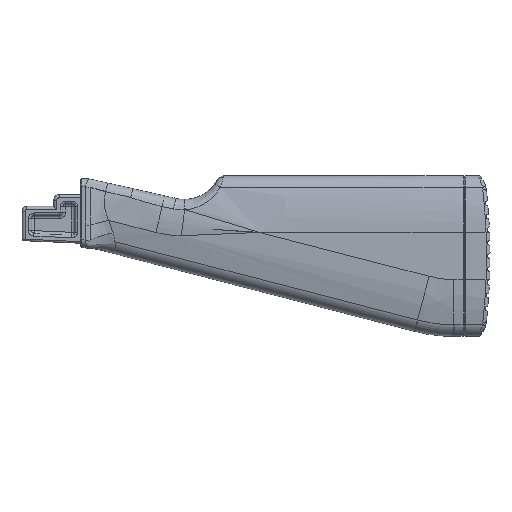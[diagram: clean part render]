
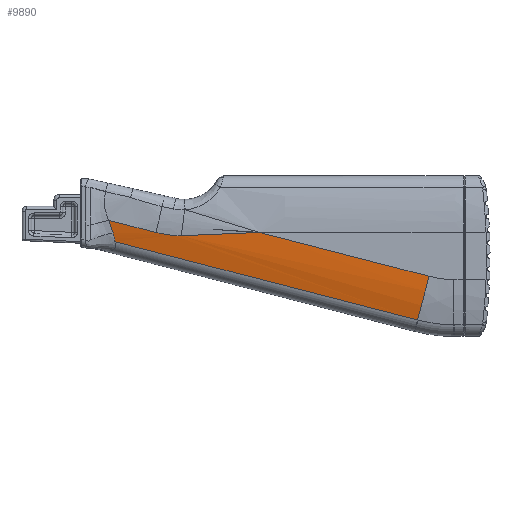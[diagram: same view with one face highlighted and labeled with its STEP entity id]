
A CAD part, left-side view. The second image highlights one B-rep face of the part: STEP entity #9890.
In plain terms, the highlighted cylindrical face has radius 115.186 mm (diameter 230.372 mm), a partial arc.
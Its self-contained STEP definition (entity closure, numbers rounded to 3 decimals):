
#368=LINE('',#16164,#820);
#514=LINE('',#30649,#966);
#820=VECTOR('',#11593,10.);
#966=VECTOR('',#12437,10.);
#1286=CYLINDRICAL_SURFACE('',#10739,115.186);
#1717=FACE_OUTER_BOUND('',#2382,.T.);
#2382=EDGE_LOOP('',(#7627,#7628,#7629,#7630,#7631,#7632,#7633,#7634,#7635));
#3047=CIRCLE('',#10731,115.186);
#3555=B_SPLINE_CURVE_WITH_KNOTS('',3,(#23032,#23033,#23034,#23035),
 .UNSPECIFIED.,.F.,.F.,(4,4),(5.073,6.041),
 .UNSPECIFIED.);
#3563=B_SPLINE_CURVE_WITH_KNOTS('',3,(#28936,#28937,#28938,#28939,#28940,
#28941),.UNSPECIFIED.,.F.,.F.,(4,2,4),(-12.142,-11.833,
-11.448),.UNSPECIFIED.);
#3585=B_SPLINE_CURVE_WITH_KNOTS('',3,(#30715,#30716,#30717,#30718),
 .UNSPECIFIED.,.F.,.F.,(4,4),(6.477,7.8),
 .UNSPECIFIED.);
#3586=B_SPLINE_CURVE_WITH_KNOTS('',3,(#30719,#30720,#30721,#30722),
 .UNSPECIFIED.,.F.,.F.,(4,4),(7.8,9.601),
 .UNSPECIFIED.);
#3587=B_SPLINE_CURVE_WITH_KNOTS('',3,(#30724,#30725,#30726,#30727,#30728,
#30729,#30730,#30731,#30732,#30733,#30734),.UNSPECIFIED.,.F.,.F.,(4,2,1,
1,1,1,1,4),(0.,0.006,0.975,
2.912,3.396,3.88,4.364,4.849),
 .UNSPECIFIED.);
#3588=B_SPLINE_CURVE_WITH_KNOTS('',3,(#30735,#30736,#30737,#30738,#30739,
#30740,#30741,#30742,#30743,#30744,#30745,#30746,#30747,#30748,#30749,#30750,
#30751,#30752,#30753,#30754,#30755,#30756,#30757),.UNSPECIFIED.,.F.,.F.,
(4,1,1,1,1,1,1,1,1,1,1,1,1,1,1,1,1,1,1,1,4),(4.849,4.888,
5.11,5.221,5.277,5.332,5.401,
5.459,5.518,5.576,5.635,5.694,
5.752,5.811,5.869,5.928,5.987,
6.045,6.158,6.265,6.477),
 .UNSPECIFIED.);
#3935=VERTEX_POINT('',#16161);
#3936=VERTEX_POINT('',#16163);
#4181=VERTEX_POINT('',#23029);
#4182=VERTEX_POINT('',#23031);
#4264=VERTEX_POINT('',#28923);
#4278=VERTEX_POINT('',#30640);
#4283=VERTEX_POINT('',#30713);
#4284=VERTEX_POINT('',#30714);
#4285=VERTEX_POINT('',#30723);
#4897=EDGE_CURVE('',#3936,#3935,#368,.T.);
#5303=EDGE_CURVE('',#4182,#4181,#3555,.T.);
#5439=EDGE_CURVE('',#4181,#4264,#3563,.T.);
#5468=EDGE_CURVE('',#4278,#3936,#3047,.T.);
#5469=EDGE_CURVE('',#4278,#4264,#514,.T.);
#5477=EDGE_CURVE('',#4283,#4284,#3585,.T.);
#5478=EDGE_CURVE('',#4284,#4182,#3586,.T.);
#5479=EDGE_CURVE('',#3935,#4285,#3587,.T.);
#5480=EDGE_CURVE('',#4285,#4283,#3588,.T.);
#7627=ORIENTED_EDGE('',*,*,#5477,.T.);
#7628=ORIENTED_EDGE('',*,*,#5478,.T.);
#7629=ORIENTED_EDGE('',*,*,#5303,.T.);
#7630=ORIENTED_EDGE('',*,*,#5439,.T.);
#7631=ORIENTED_EDGE('',*,*,#5469,.F.);
#7632=ORIENTED_EDGE('',*,*,#5468,.T.);
#7633=ORIENTED_EDGE('',*,*,#4897,.T.);
#7634=ORIENTED_EDGE('',*,*,#5479,.T.);
#7635=ORIENTED_EDGE('',*,*,#5480,.T.);
#9890=ADVANCED_FACE('',(#1717),#1286,.T.);
#10731=AXIS2_PLACEMENT_3D('',#30647,#12433,#12434);
#10739=AXIS2_PLACEMENT_3D('',#30712,#12451,#12452);
#11593=DIRECTION('',(0.,0.968,0.25));
#12433=DIRECTION('center_axis',(0.,0.967,0.253));
#12434=DIRECTION('ref_axis',(-0.949,0.08,-0.305));
#12437=DIRECTION('',(0.,0.968,0.25));
#12451=DIRECTION('center_axis',(0.,-0.968,-0.25));
#12452=DIRECTION('ref_axis',(-0.949,0.079,-0.305));
#16161=CARTESIAN_POINT('',(84.25,-573.566,96.326));
#16163=CARTESIAN_POINT('',(84.25,-681.487,68.407));
#16164=CARTESIAN_POINT('',(84.25,-681.381,68.434));
#23029=CARTESIAN_POINT('',(86.683,-480.14,96.168));
#23031=CARTESIAN_POINT('',(85.452,-477.378,104.065));
#23032=CARTESIAN_POINT('Ctrl Pts',(85.452,-477.378,104.065));
#23033=CARTESIAN_POINT('Ctrl Pts',(85.795,-478.261,101.405));
#23034=CARTESIAN_POINT('Ctrl Pts',(86.207,-479.2,98.766));
#23035=CARTESIAN_POINT('Ctrl Pts',(86.683,-480.14,96.168));
#28923=CARTESIAN_POINT('',(87.904,-481.18,90.497));
#28936=CARTESIAN_POINT('Ctrl Pts',(86.683,-480.14,96.168));
#28937=CARTESIAN_POINT('Ctrl Pts',(86.836,-480.441,95.337));
#28938=CARTESIAN_POINT('Ctrl Pts',(87.002,-480.676,94.493));
#28939=CARTESIAN_POINT('Ctrl Pts',(87.403,-481.058,92.592));
#28940=CARTESIAN_POINT('Ctrl Pts',(87.645,-481.168,91.535));
#28941=CARTESIAN_POINT('Ctrl Pts',(87.904,-481.18,90.497));
#30640=CARTESIAN_POINT('',(87.904,-674.191,40.564));
#30647=CARTESIAN_POINT('Origin',(199.436,-681.487,68.406));
#30649=CARTESIAN_POINT('',(87.904,-530.082,77.846));
#30712=CARTESIAN_POINT('Origin',(199.436,-681.381,68.434));
#30713=CARTESIAN_POINT('',(85.443,-507.458,96.349));
#30714=CARTESIAN_POINT('',(85.447,-494.719,99.616));
#30715=CARTESIAN_POINT('Ctrl Pts',(85.443,-507.458,96.349));
#30716=CARTESIAN_POINT('Ctrl Pts',(85.444,-503.212,97.438));
#30717=CARTESIAN_POINT('Ctrl Pts',(85.446,-498.966,98.526));
#30718=CARTESIAN_POINT('Ctrl Pts',(85.447,-494.719,99.616));
#30719=CARTESIAN_POINT('Ctrl Pts',(85.447,-494.719,99.616));
#30720=CARTESIAN_POINT('Ctrl Pts',(85.449,-488.939,101.098));
#30721=CARTESIAN_POINT('Ctrl Pts',(85.451,-483.159,102.581));
#30722=CARTESIAN_POINT('Ctrl Pts',(85.452,-477.378,104.065));
#30723=CARTESIAN_POINT('',(85.166,-523.604,94.277));
#30724=CARTESIAN_POINT('Ctrl Pts',(84.25,-573.566,96.326));
#30725=CARTESIAN_POINT('Ctrl Pts',(84.25,-573.545,96.324));
#30726=CARTESIAN_POINT('Ctrl Pts',(84.25,-573.525,96.323));
#30727=CARTESIAN_POINT('Ctrl Pts',(84.25,-570.15,96.073));
#30728=CARTESIAN_POINT('Ctrl Pts',(84.296,-560.108,95.403));
#30729=CARTESIAN_POINT('Ctrl Pts',(84.488,-548.453,94.866));
#30730=CARTESIAN_POINT('Ctrl Pts',(84.726,-538.492,94.559));
#30731=CARTESIAN_POINT('Ctrl Pts',(84.859,-533.528,94.436));
#30732=CARTESIAN_POINT('Ctrl Pts',(85.006,-528.546,94.34));
#30733=CARTESIAN_POINT('Ctrl Pts',(85.111,-525.267,94.296));
#30734=CARTESIAN_POINT('Ctrl Pts',(85.166,-523.604,94.277));
#30735=CARTESIAN_POINT('Ctrl Pts',(85.166,-523.604,94.277));
#30736=CARTESIAN_POINT('Ctrl Pts',(85.17,-523.468,94.276));
#30737=CARTESIAN_POINT('Ctrl Pts',(85.2,-522.567,94.269));
#30738=CARTESIAN_POINT('Ctrl Pts',(85.238,-521.315,94.293));
#30739=CARTESIAN_POINT('Ctrl Pts',(85.274,-520.004,94.355));
#30740=CARTESIAN_POINT('Ctrl Pts',(85.293,-519.242,94.403));
#30741=CARTESIAN_POINT('Ctrl Pts',(85.307,-518.681,94.445));
#30742=CARTESIAN_POINT('Ctrl Pts',(85.322,-518.052,94.497));
#30743=CARTESIAN_POINT('Ctrl Pts',(85.335,-517.441,94.555));
#30744=CARTESIAN_POINT('Ctrl Pts',(85.347,-516.853,94.616));
#30745=CARTESIAN_POINT('Ctrl Pts',(85.358,-516.271,94.682));
#30746=CARTESIAN_POINT('Ctrl Pts',(85.369,-515.688,94.754));
#30747=CARTESIAN_POINT('Ctrl Pts',(85.379,-515.107,94.832));
#30748=CARTESIAN_POINT('Ctrl Pts',(85.388,-514.527,94.914));
#30749=CARTESIAN_POINT('Ctrl Pts',(85.397,-513.948,95.003));
#30750=CARTESIAN_POINT('Ctrl Pts',(85.404,-513.371,95.096));
#30751=CARTESIAN_POINT('Ctrl Pts',(85.411,-512.795,95.194));
#30752=CARTESIAN_POINT('Ctrl Pts',(85.418,-512.22,95.297));
#30753=CARTESIAN_POINT('Ctrl Pts',(85.425,-511.469,95.439));
#30754=CARTESIAN_POINT('Ctrl Pts',(85.432,-510.563,95.622));
#30755=CARTESIAN_POINT('Ctrl Pts',(85.44,-509.167,95.927));
#30756=CARTESIAN_POINT('Ctrl Pts',(85.443,-508.138,96.175));
#30757=CARTESIAN_POINT('Ctrl Pts',(85.443,-507.458,96.349));
